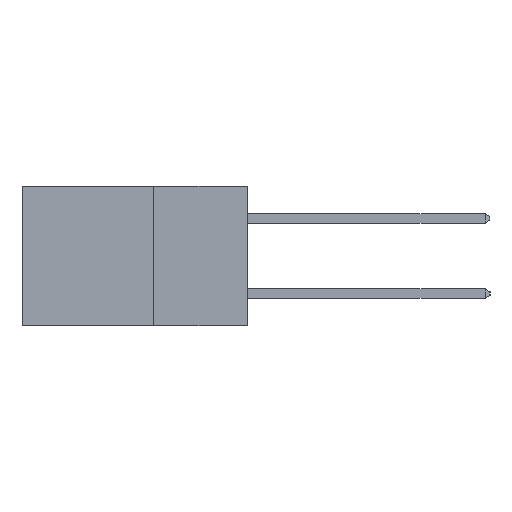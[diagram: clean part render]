
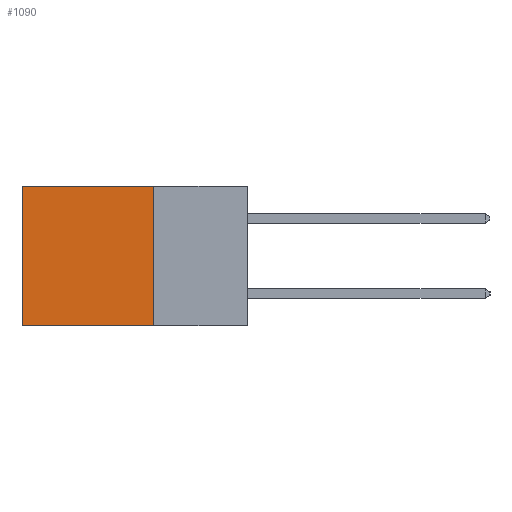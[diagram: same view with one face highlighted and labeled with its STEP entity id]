
A CAD part, left-side view. The second image highlights one B-rep face of the part: STEP entity #1090.
In plain terms, the highlighted planar face has unit normal (-1, 0, 0).
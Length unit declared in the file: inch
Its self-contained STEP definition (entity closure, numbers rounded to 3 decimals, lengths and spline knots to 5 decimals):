
#201 = VECTOR ( 'NONE', #3679, 39.37008 ) ;
#1090 = ADVANCED_FACE ( 'NONE', ( #1519 ), #8772, .F. ) ;
#1190 = EDGE_CURVE ( 'NONE', #14756, #13119, #3406, .T. ) ;
#1519 = FACE_OUTER_BOUND ( 'NONE', #8671, .T. ) ;
#1523 = CARTESIAN_POINT ( 'NONE',  ( 0.2615, 0.6, -0.37 ) ) ;
#2431 = ORIENTED_EDGE ( 'NONE', *, *, #1190, .F. ) ;
#2675 = VERTEX_POINT ( 'NONE', #5567 ) ;
#3406 = LINE ( 'NONE', #7076, #201 ) ;
#3521 = LINE ( 'NONE', #15610, #13329 ) ;
#3561 = ORIENTED_EDGE ( 'NONE', *, *, #16939, .F. ) ;
#3679 = DIRECTION ( 'NONE',  ( 0., 1., 0. ) ) ;
#5025 = VERTEX_POINT ( 'NONE', #13831 ) ;
#5533 = DIRECTION ( 'NONE',  ( 0., 0., -1. ) ) ;
#5567 = CARTESIAN_POINT ( 'NONE',  ( 0.2615, 0.25, 0. ) ) ;
#7076 = CARTESIAN_POINT ( 'NONE',  ( 0.2615, 0.25, -0.37 ) ) ;
#8671 = EDGE_LOOP ( 'NONE', ( #12834, #2431, #3561, #9433 ) ) ;
#8772 = PLANE ( 'NONE',  #13265 ) ;
#9433 = ORIENTED_EDGE ( 'NONE', *, *, #10559, .T. ) ;
#9468 = CARTESIAN_POINT ( 'NONE',  ( 0.2615, 0.6, -0.37 ) ) ;
#9568 = DIRECTION ( 'NONE',  ( 1., 0., 0. ) ) ;
#10222 = LINE ( 'NONE', #11055, #16846 ) ;
#10559 = EDGE_CURVE ( 'NONE', #2675, #5025, #10222, .T. ) ;
#10778 = DIRECTION ( 'NONE',  ( 0., 1., 0. ) ) ;
#11055 = CARTESIAN_POINT ( 'NONE',  ( 0.2615, 0.25, 0. ) ) ;
#11106 = EDGE_CURVE ( 'NONE', #5025, #13119, #12523, .T. ) ;
#11601 = DIRECTION ( 'NONE',  ( 0., 0., -1. ) ) ;
#12523 = LINE ( 'NONE', #1523, #15627 ) ;
#12834 = ORIENTED_EDGE ( 'NONE', *, *, #11106, .T. ) ;
#13119 = VERTEX_POINT ( 'NONE', #9468 ) ;
#13265 = AXIS2_PLACEMENT_3D ( 'NONE', #13637, #9568, #5533 ) ;
#13329 = VECTOR ( 'NONE', #11601, 39.37008 ) ;
#13551 = DIRECTION ( 'NONE',  ( 0., 0., -1. ) ) ;
#13637 = CARTESIAN_POINT ( 'NONE',  ( 0.2615, 0.25, -0.37 ) ) ;
#13831 = CARTESIAN_POINT ( 'NONE',  ( 0.2615, 0.6, 0. ) ) ;
#14756 = VERTEX_POINT ( 'NONE', #16036 ) ;
#15610 = CARTESIAN_POINT ( 'NONE',  ( 0.2615, 0.25, -0.37 ) ) ;
#15627 = VECTOR ( 'NONE', #13551, 39.37008 ) ;
#16036 = CARTESIAN_POINT ( 'NONE',  ( 0.2615, 0.25, -0.37 ) ) ;
#16846 = VECTOR ( 'NONE', #10778, 39.37008 ) ;
#16939 = EDGE_CURVE ( 'NONE', #2675, #14756, #3521, .T. ) ;
